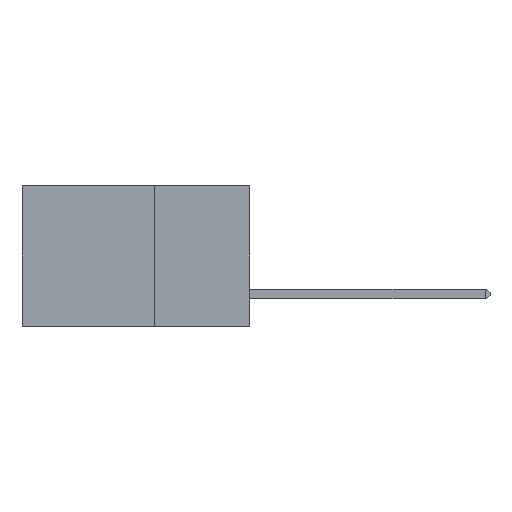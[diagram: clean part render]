
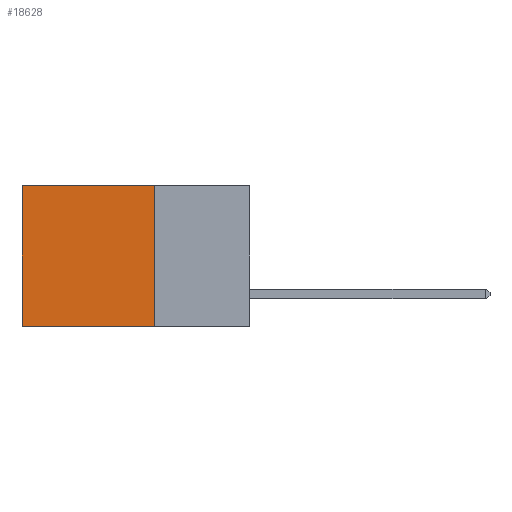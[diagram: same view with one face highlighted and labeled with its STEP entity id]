
A CAD part, left-side view. The second image highlights one B-rep face of the part: STEP entity #18628.
In plain terms, the highlighted planar face has unit normal (-1, 0, 0).
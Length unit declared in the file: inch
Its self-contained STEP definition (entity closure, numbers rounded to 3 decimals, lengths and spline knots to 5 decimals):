
#310 = ORIENTED_EDGE ( 'NONE', *, *, #18574, .F. ) ;
#528 = DIRECTION ( 'NONE',  ( 0., 0., -1. ) ) ;
#716 = CARTESIAN_POINT ( 'NONE',  ( 0.2875, 0.25, 0. ) ) ;
#1137 = VECTOR ( 'NONE', #3388, 39.37008 ) ;
#1752 = ORIENTED_EDGE ( 'NONE', *, *, #8154, .T. ) ;
#3388 = DIRECTION ( 'NONE',  ( 0., 1., 0. ) ) ;
#3603 = CARTESIAN_POINT ( 'NONE',  ( 0.2875, 0.25, 0. ) ) ;
#4807 = CARTESIAN_POINT ( 'NONE',  ( 0.2875, 0.6, 0. ) ) ;
#5402 = VECTOR ( 'NONE', #528, 39.37008 ) ;
#7101 = LINE ( 'NONE', #13673, #12437 ) ;
#8103 = LINE ( 'NONE', #716, #1137 ) ;
#8154 = EDGE_CURVE ( 'NONE', #10538, #14662, #8103, .T. ) ;
#8861 = PLANE ( 'NONE',  #12695 ) ;
#10538 = VERTEX_POINT ( 'NONE', #18438 ) ;
#11398 = CARTESIAN_POINT ( 'NONE',  ( 0.2875, 0.6, 0. ) ) ;
#12437 = VECTOR ( 'NONE', #18925, 39.37008 ) ;
#12695 = AXIS2_PLACEMENT_3D ( 'NONE', #3603, #14100, #31976 ) ;
#13673 = CARTESIAN_POINT ( 'NONE',  ( 0.2875, 0.25, -0.37 ) ) ;
#14100 = DIRECTION ( 'NONE',  ( 1., 0., 0. ) ) ;
#14662 = VERTEX_POINT ( 'NONE', #11398 ) ;
#15780 = VERTEX_POINT ( 'NONE', #31502 ) ;
#18438 = CARTESIAN_POINT ( 'NONE',  ( 0.2875, 0.25, 0. ) ) ;
#18574 = EDGE_CURVE ( 'NONE', #31259, #15780, #7101, .T. ) ;
#18628 = ADVANCED_FACE ( 'NONE', ( #32066 ), #8861, .F. ) ;
#18925 = DIRECTION ( 'NONE',  ( 0., 1., 0. ) ) ;
#22500 = EDGE_LOOP ( 'NONE', ( #23036, #310, #29902, #1752 ) ) ;
#23036 = ORIENTED_EDGE ( 'NONE', *, *, #33254, .T. ) ;
#25568 = DIRECTION ( 'NONE',  ( 0., 0., -1. ) ) ;
#26102 = LINE ( 'NONE', #31500, #5402 ) ;
#26322 = VECTOR ( 'NONE', #25568, 39.37008 ) ;
#29409 = CARTESIAN_POINT ( 'NONE',  ( 0.2875, 0.25, -0.37 ) ) ;
#29902 = ORIENTED_EDGE ( 'NONE', *, *, #31168, .F. ) ;
#31168 = EDGE_CURVE ( 'NONE', #10538, #31259, #26102, .T. ) ;
#31259 = VERTEX_POINT ( 'NONE', #29409 ) ;
#31500 = CARTESIAN_POINT ( 'NONE',  ( 0.2875, 0.25, 0. ) ) ;
#31502 = CARTESIAN_POINT ( 'NONE',  ( 0.2875, 0.6, -0.37 ) ) ;
#31976 = DIRECTION ( 'NONE',  ( 0., 0., -1. ) ) ;
#32066 = FACE_OUTER_BOUND ( 'NONE', #22500, .T. ) ;
#32223 = LINE ( 'NONE', #4807, #26322 ) ;
#33254 = EDGE_CURVE ( 'NONE', #14662, #15780, #32223, .T. ) ;
